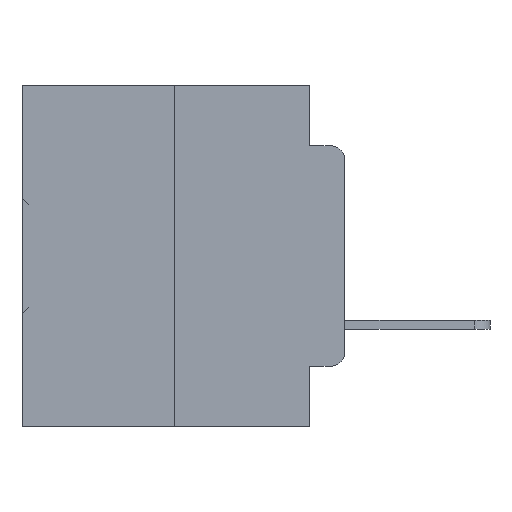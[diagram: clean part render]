
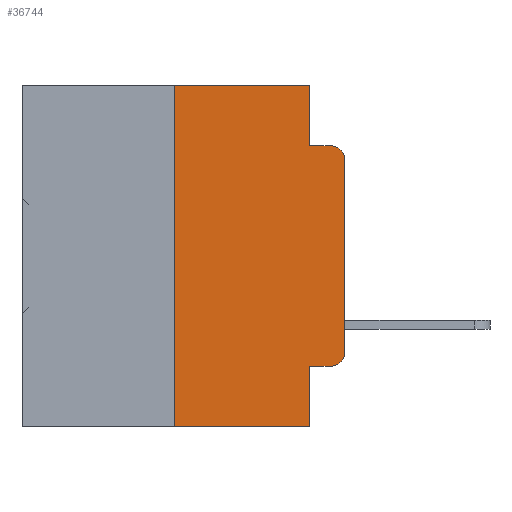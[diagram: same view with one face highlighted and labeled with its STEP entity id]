
A CAD part, left-side view. The second image highlights one B-rep face of the part: STEP entity #36744.
In plain terms, the highlighted planar face has unit normal (-1, 0, 0).
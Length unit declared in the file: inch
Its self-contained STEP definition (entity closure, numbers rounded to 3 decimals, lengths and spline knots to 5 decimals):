
#80 = VERTEX_POINT ( 'NONE', #35354 ) ;
#730 = VECTOR ( 'NONE', #1773, 39.37008 ) ;
#950 = CARTESIAN_POINT ( 'NONE',  ( 0., 0.25, -0.5 ) ) ;
#1327 = VECTOR ( 'NONE', #30073, 39.37008 ) ;
#1698 = LINE ( 'NONE', #19167, #730 ) ;
#1773 = DIRECTION ( 'NONE',  ( 0., -1., 0. ) ) ;
#2152 = FACE_OUTER_BOUND ( 'NONE', #17603, .T. ) ;
#2630 = ORIENTED_EDGE ( 'NONE', *, *, #28841, .T. ) ;
#2677 = LINE ( 'NONE', #35484, #13213 ) ;
#3339 = DIRECTION ( 'NONE',  ( 0., -1., 0. ) ) ;
#4454 = CARTESIAN_POINT ( 'NONE',  ( 0., 0., 0. ) ) ;
#4509 = ORIENTED_EDGE ( 'NONE', *, *, #15811, .T. ) ;
#4800 = CARTESIAN_POINT ( 'NONE',  ( 0., 0.051, 0. ) ) ;
#5415 = AXIS2_PLACEMENT_3D ( 'NONE', #26677, #9760, #29472 ) ;
#5566 = ORIENTED_EDGE ( 'NONE', *, *, #30252, .T. ) ;
#5758 = VERTEX_POINT ( 'NONE', #22376 ) ;
#6562 = LINE ( 'NONE', #4800, #7478 ) ;
#6805 = EDGE_CURVE ( 'NONE', #28013, #19139, #2677, .T. ) ;
#6959 = LINE ( 'NONE', #17750, #35189 ) ;
#7478 = VECTOR ( 'NONE', #13546, 39.37008 ) ;
#7752 = CARTESIAN_POINT ( 'NONE',  ( 0., 0.051, 0. ) ) ;
#8007 = EDGE_CURVE ( 'NONE', #28157, #18509, #1698, .T. ) ;
#9110 = CIRCLE ( 'NONE', #5415, 0.02 ) ;
#9760 = DIRECTION ( 'NONE',  ( -1., 0., 0. ) ) ;
#10041 = ORIENTED_EDGE ( 'NONE', *, *, #8007, .F. ) ;
#10070 = DIRECTION ( 'NONE',  ( -1., 0., 0. ) ) ;
#11617 = CARTESIAN_POINT ( 'NONE',  ( 0., 0.473, 0. ) ) ;
#11737 = DIRECTION ( 'NONE',  ( 0., 0., -1. ) ) ;
#11995 = DIRECTION ( 'NONE',  ( 0., 0., 1. ) ) ;
#12740 = AXIS2_PLACEMENT_3D ( 'NONE', #11617, #28593, #11737 ) ;
#13213 = VECTOR ( 'NONE', #13289, 39.37008 ) ;
#13289 = DIRECTION ( 'NONE',  ( 0., 0., -1. ) ) ;
#13546 = DIRECTION ( 'NONE',  ( 0., 0., -1. ) ) ;
#15659 = ORIENTED_EDGE ( 'NONE', *, *, #28372, .T. ) ;
#15712 = CARTESIAN_POINT ( 'NONE',  ( 0., 0.051, -0.5 ) ) ;
#15811 = EDGE_CURVE ( 'NONE', #25792, #19139, #25316, .T. ) ;
#16005 = CARTESIAN_POINT ( 'NONE',  ( 0., 0.02, -0.4115 ) ) ;
#17005 = VECTOR ( 'NONE', #27529, 39.37008 ) ;
#17090 = CARTESIAN_POINT ( 'NONE',  ( 0., 0.25, 0. ) ) ;
#17603 = EDGE_LOOP ( 'NONE', ( #2630, #25100, #35554, #26869, #10041, #28978, #4509, #30414, #5566, #15659 ) ) ;
#17621 = VECTOR ( 'NONE', #26165, 39.37008 ) ;
#17717 = VECTOR ( 'NONE', #3339, 39.37008 ) ;
#17750 = CARTESIAN_POINT ( 'NONE',  ( 0., 0.25, 0. ) ) ;
#18509 = VERTEX_POINT ( 'NONE', #7752 ) ;
#19139 = VERTEX_POINT ( 'NONE', #15712 ) ;
#19167 = CARTESIAN_POINT ( 'NONE',  ( 0., 0.473, 0. ) ) ;
#20208 = EDGE_CURVE ( 'NONE', #25792, #28157, #6959, .T. ) ;
#20614 = AXIS2_PLACEMENT_3D ( 'NONE', #26988, #10070, #29789 ) ;
#22103 = CARTESIAN_POINT ( 'NONE',  ( 0., 0.051, -0.4115 ) ) ;
#22376 = CARTESIAN_POINT ( 'NONE',  ( 0., 0.02, -0.0885 ) ) ;
#22972 = PLANE ( 'NONE',  #12740 ) ;
#23414 = CARTESIAN_POINT ( 'NONE',  ( 0., 0.051, -0.4115 ) ) ;
#23981 = VERTEX_POINT ( 'NONE', #33316 ) ;
#24715 = CARTESIAN_POINT ( 'NONE',  ( 0., 0.473, -0.5 ) ) ;
#25054 = LINE ( 'NONE', #31779, #17621 ) ;
#25100 = ORIENTED_EDGE ( 'NONE', *, *, #25116, .T. ) ;
#25116 = EDGE_CURVE ( 'NONE', #36193, #5758, #9110, .T. ) ;
#25153 = LINE ( 'NONE', #23414, #17717 ) ;
#25211 = LINE ( 'NONE', #4454, #1327 ) ;
#25316 = LINE ( 'NONE', #24715, #17005 ) ;
#25792 = VERTEX_POINT ( 'NONE', #950 ) ;
#26165 = DIRECTION ( 'NONE',  ( 0., -1., 0. ) ) ;
#26677 = CARTESIAN_POINT ( 'NONE',  ( 0., 0.02, -0.1085 ) ) ;
#26869 = ORIENTED_EDGE ( 'NONE', *, *, #29560, .F. ) ;
#26988 = CARTESIAN_POINT ( 'NONE',  ( 0., 0.02, -0.3915 ) ) ;
#27013 = CIRCLE ( 'NONE', #20614, 0.02 ) ;
#27529 = DIRECTION ( 'NONE',  ( 0., -1., 0. ) ) ;
#28013 = VERTEX_POINT ( 'NONE', #22103 ) ;
#28157 = VERTEX_POINT ( 'NONE', #17090 ) ;
#28372 = EDGE_CURVE ( 'NONE', #34577, #23981, #27013, .T. ) ;
#28593 = DIRECTION ( 'NONE',  ( 1., 0., 0. ) ) ;
#28841 = EDGE_CURVE ( 'NONE', #23981, #36193, #25211, .T. ) ;
#28978 = ORIENTED_EDGE ( 'NONE', *, *, #20208, .F. ) ;
#29472 = DIRECTION ( 'NONE',  ( 0., 0., -1. ) ) ;
#29560 = EDGE_CURVE ( 'NONE', #18509, #80, #6562, .T. ) ;
#29789 = DIRECTION ( 'NONE',  ( 0., 0., -1. ) ) ;
#30073 = DIRECTION ( 'NONE',  ( 0., 0., 1. ) ) ;
#30252 = EDGE_CURVE ( 'NONE', #28013, #34577, #25153, .T. ) ;
#30414 = ORIENTED_EDGE ( 'NONE', *, *, #6805, .F. ) ;
#31565 = CARTESIAN_POINT ( 'NONE',  ( 0., 0., -0.1085 ) ) ;
#31779 = CARTESIAN_POINT ( 'NONE',  ( 0., 0.051, -0.0885 ) ) ;
#33316 = CARTESIAN_POINT ( 'NONE',  ( 0., 0., -0.3915 ) ) ;
#33317 = EDGE_CURVE ( 'NONE', #80, #5758, #25054, .T. ) ;
#34577 = VERTEX_POINT ( 'NONE', #16005 ) ;
#35189 = VECTOR ( 'NONE', #11995, 39.37008 ) ;
#35354 = CARTESIAN_POINT ( 'NONE',  ( 0., 0.051, -0.0885 ) ) ;
#35484 = CARTESIAN_POINT ( 'NONE',  ( 0., 0.051, 0. ) ) ;
#35554 = ORIENTED_EDGE ( 'NONE', *, *, #33317, .F. ) ;
#36193 = VERTEX_POINT ( 'NONE', #31565 ) ;
#36744 = ADVANCED_FACE ( 'NONE', ( #2152 ), #22972, .F. ) ;
